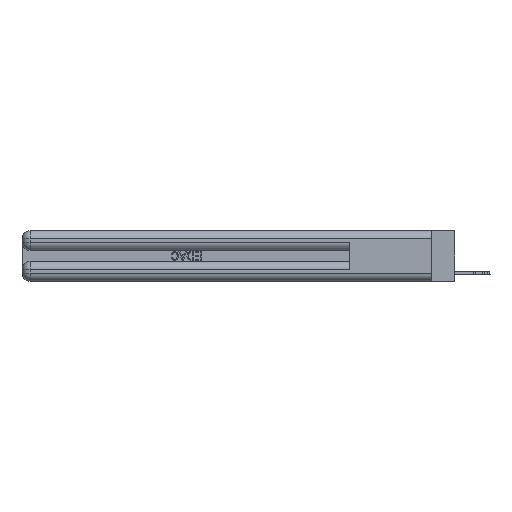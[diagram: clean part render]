
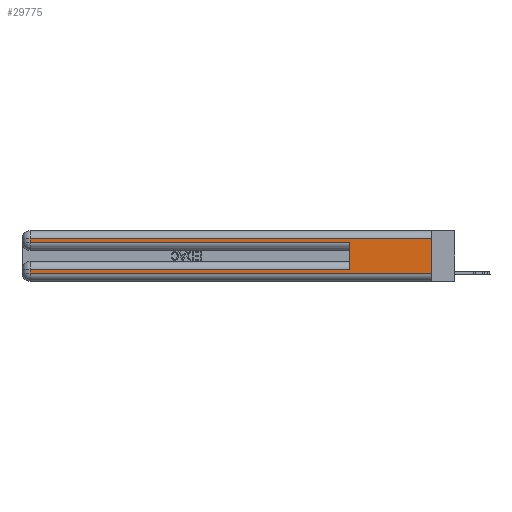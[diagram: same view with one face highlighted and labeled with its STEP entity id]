
A CAD part, left-side view. The second image highlights one B-rep face of the part: STEP entity #29775.
In plain terms, the highlighted planar face has unit normal (-1, 0, 0).
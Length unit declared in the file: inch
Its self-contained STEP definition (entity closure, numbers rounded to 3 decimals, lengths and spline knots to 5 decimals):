
#162 = ORIENTED_EDGE ( 'NONE', *, *, #7499, .T. ) ;
#276 = CARTESIAN_POINT ( 'NONE',  ( 0., 2.94, 0.31 ) ) ;
#289 = LINE ( 'NONE', #28560, #10875 ) ;
#380 = EDGE_CURVE ( 'NONE', #23087, #867, #289, .T. ) ;
#595 = AXIS2_PLACEMENT_3D ( 'NONE', #26293, #3549, #23405 ) ;
#867 = VERTEX_POINT ( 'NONE', #7235 ) ;
#1027 = ORIENTED_EDGE ( 'NONE', *, *, #4015, .T. ) ;
#1396 = VERTEX_POINT ( 'NONE', #30073 ) ;
#2146 = ORIENTED_EDGE ( 'NONE', *, *, #380, .T. ) ;
#2152 = VERTEX_POINT ( 'NONE', #8981 ) ;
#2297 = CARTESIAN_POINT ( 'NONE',  ( 0., 0.6, 0.085 ) ) ;
#2493 = CARTESIAN_POINT ( 'NONE',  ( 0., 2.94, 0.285 ) ) ;
#2888 = DIRECTION ( 'NONE',  ( 0., 0., -1. ) ) ;
#3470 = VERTEX_POINT ( 'NONE', #24128 ) ;
#3549 = DIRECTION ( 'NONE',  ( 1., 0., 0. ) ) ;
#3604 = CARTESIAN_POINT ( 'NONE',  ( 0., 0., 0.285 ) ) ;
#4015 = EDGE_CURVE ( 'NONE', #2152, #31522, #30017, .T. ) ;
#5063 = CARTESIAN_POINT ( 'NONE',  ( 0., 2.94, 0.37 ) ) ;
#5668 = DIRECTION ( 'NONE',  ( 0., 1., 0. ) ) ;
#7235 = CARTESIAN_POINT ( 'NONE',  ( 0., 2.94, 0.085 ) ) ;
#7499 = EDGE_CURVE ( 'NONE', #7766, #3470, #25113, .T. ) ;
#7766 = VERTEX_POINT ( 'NONE', #2493 ) ;
#8338 = DIRECTION ( 'NONE',  ( 0., -1., 0. ) ) ;
#8343 = EDGE_CURVE ( 'NONE', #10470, #1396, #11485, .T. ) ;
#8570 = VECTOR ( 'NONE', #25027, 39.37008 ) ;
#8981 = CARTESIAN_POINT ( 'NONE',  ( 0., 0., 0.31 ) ) ;
#10470 = VERTEX_POINT ( 'NONE', #32130 ) ;
#10875 = VECTOR ( 'NONE', #16733, 39.37008 ) ;
#10950 = CARTESIAN_POINT ( 'NONE',  ( 0., 0., 0.06 ) ) ;
#11485 = LINE ( 'NONE', #10950, #8570 ) ;
#11486 = EDGE_CURVE ( 'NONE', #23087, #3470, #25548, .T. ) ;
#12584 = VECTOR ( 'NONE', #8338, 39.37008 ) ;
#13025 = ORIENTED_EDGE ( 'NONE', *, *, #19435, .T. ) ;
#13186 = VECTOR ( 'NONE', #26262, 39.37008 ) ;
#16655 = LINE ( 'NONE', #33558, #18416 ) ;
#16733 = DIRECTION ( 'NONE',  ( 0., 1., 0. ) ) ;
#18179 = FACE_OUTER_BOUND ( 'NONE', #27589, .T. ) ;
#18416 = VECTOR ( 'NONE', #22259, 39.37008 ) ;
#19133 = DIRECTION ( 'NONE',  ( 0., 0., -1. ) ) ;
#19435 = EDGE_CURVE ( 'NONE', #31522, #7766, #22214, .T. ) ;
#19969 = ORIENTED_EDGE ( 'NONE', *, *, #8343, .T. ) ;
#22158 = VECTOR ( 'NONE', #2888, 39.37008 ) ;
#22214 = LINE ( 'NONE', #32632, #26761 ) ;
#22259 = DIRECTION ( 'NONE',  ( 0., 0., -1. ) ) ;
#23087 = VERTEX_POINT ( 'NONE', #2297 ) ;
#23405 = DIRECTION ( 'NONE',  ( 0., 0., -1. ) ) ;
#24128 = CARTESIAN_POINT ( 'NONE',  ( 0., 0.6, 0.285 ) ) ;
#24728 = LINE ( 'NONE', #5063, #22158 ) ;
#25027 = DIRECTION ( 'NONE',  ( 0., -1., 0. ) ) ;
#25113 = LINE ( 'NONE', #3604, #12584 ) ;
#25548 = LINE ( 'NONE', #28250, #13186 ) ;
#25772 = ORIENTED_EDGE ( 'NONE', *, *, #26307, .F. ) ;
#26109 = PLANE ( 'NONE',  #595 ) ;
#26262 = DIRECTION ( 'NONE',  ( 0., 0., 1. ) ) ;
#26293 = CARTESIAN_POINT ( 'NONE',  ( 0., 0., 0.37 ) ) ;
#26307 = EDGE_CURVE ( 'NONE', #2152, #1396, #16655, .T. ) ;
#26761 = VECTOR ( 'NONE', #19133, 39.37008 ) ;
#27589 = EDGE_LOOP ( 'NONE', ( #25772, #1027, #13025, #162, #29776, #2146, #31227, #19969 ) ) ;
#28250 = CARTESIAN_POINT ( 'NONE',  ( 0., 0.6, 0.145 ) ) ;
#28560 = CARTESIAN_POINT ( 'NONE',  ( 0., 0., 0.085 ) ) ;
#29775 = ADVANCED_FACE ( 'NONE', ( #18179 ), #26109, .F. ) ;
#29776 = ORIENTED_EDGE ( 'NONE', *, *, #11486, .F. ) ;
#30017 = LINE ( 'NONE', #30555, #35035 ) ;
#30073 = CARTESIAN_POINT ( 'NONE',  ( 0., 0., 0.06 ) ) ;
#30555 = CARTESIAN_POINT ( 'NONE',  ( 0., 0., 0.31 ) ) ;
#31227 = ORIENTED_EDGE ( 'NONE', *, *, #35586, .T. ) ;
#31522 = VERTEX_POINT ( 'NONE', #276 ) ;
#32130 = CARTESIAN_POINT ( 'NONE',  ( 0., 2.94, 0.06 ) ) ;
#32632 = CARTESIAN_POINT ( 'NONE',  ( 0., 2.94, 0.37 ) ) ;
#33558 = CARTESIAN_POINT ( 'NONE',  ( 0., 0., 0.37 ) ) ;
#35035 = VECTOR ( 'NONE', #5668, 39.37008 ) ;
#35586 = EDGE_CURVE ( 'NONE', #867, #10470, #24728, .T. ) ;
